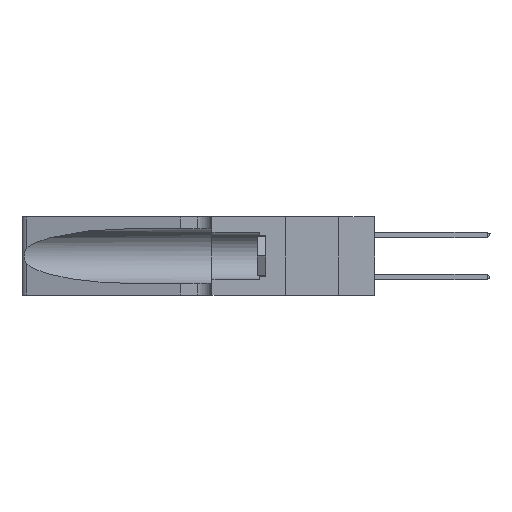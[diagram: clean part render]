
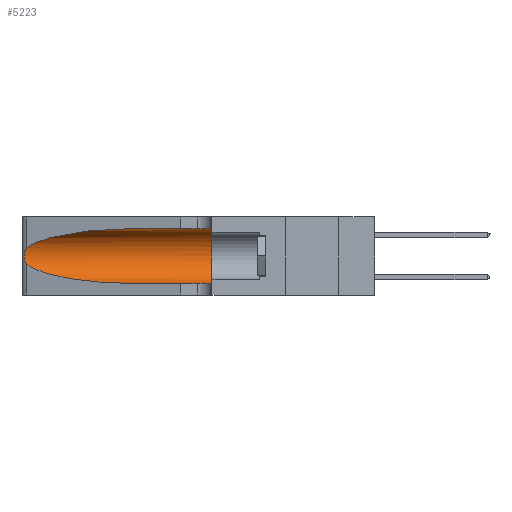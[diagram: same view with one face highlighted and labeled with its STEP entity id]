
A CAD part, left-side view. The second image highlights one B-rep face of the part: STEP entity #5223.
In plain terms, the highlighted cylindrical face has radius 3.308 mm (diameter 6.617 mm), a partial arc.
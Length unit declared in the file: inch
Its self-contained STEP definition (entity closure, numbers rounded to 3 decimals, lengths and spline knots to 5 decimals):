
#881 = CARTESIAN_POINT ( 'NONE',  ( 0.1305, 1.61858, 0.05475 ) ) ;
#1154 = EDGE_CURVE ( 'NONE', #2399, #32130, #8456, .T. ) ;
#1244 = ORIENTED_EDGE ( 'NONE', *, *, #23705, .T. ) ;
#1579 =( BOUNDED_CURVE ( )  B_SPLINE_CURVE ( 3, ( #5266, #29837, #29720, #38854 ),
 .UNSPECIFIED., .F., .F. ) 
 B_SPLINE_CURVE_WITH_KNOTS ( ( 4, 4 ),
 ( 1.5708, 2.84003 ),
 .UNSPECIFIED. ) 
 CURVE ( )  GEOMETRIC_REPRESENTATION_ITEM ( )  RATIONAL_B_SPLINE_CURVE ( ( 1., 0.87, 0.87, 1. ) ) 
 REPRESENTATION_ITEM ( '' )  );
#1945 = CARTESIAN_POINT ( 'NONE',  ( 0.26018, 1.23835, 0.19895 ) ) ;
#2399 = VERTEX_POINT ( 'NONE', #8929 ) ;
#2957 = ORIENTED_EDGE ( 'NONE', *, *, #26827, .T. ) ;
#3782 = EDGE_CURVE ( 'NONE', #24122, #13965, #1579, .T. ) ;
#3819 = VERTEX_POINT ( 'NONE', #29174 ) ;
#4473 = DIRECTION ( 'NONE',  ( 0., -1., 0. ) ) ;
#5223 = ADVANCED_FACE ( 'NONE', ( #20874 ), #28402, .F. ) ;
#5266 = CARTESIAN_POINT ( 'NONE',  ( 0.1305, 0.72297, 0.31525 ) ) ;
#5659 = CARTESIAN_POINT ( 'NONE',  ( 0.2373, 1.15595, 0.08982 ) ) ;
#6917 = DIRECTION ( 'NONE',  ( 0., 1., 0. ) ) ;
#7857 = VECTOR ( 'NONE', #20168, 39.37008 ) ;
#7904 = CARTESIAN_POINT ( 'NONE',  ( 0.26075, 1.23896, 0.178 ) ) ;
#8456 = CIRCLE ( 'NONE', #23205, 0.13025 ) ;
#8870 = CARTESIAN_POINT ( 'NONE',  ( 0.25487, 1.22718, 0.14631 ) ) ;
#8929 = CARTESIAN_POINT ( 'NONE',  ( 0.1305, 0.35, 0.31525 ) ) ;
#9087 = CARTESIAN_POINT ( 'NONE',  ( 0.1305, 0.72297, 0.05475 ) ) ;
#9824 = B_SPLINE_CURVE_WITH_KNOTS ( 'NONE', 3,
 ( #29441, #16912, #25865, #32092, #11217, #1945, #26258, #7904, #38062, #14008, #14292, #17045, #35158, #17284 ),
 .UNSPECIFIED., .F., .F.,
 ( 4, 2, 2, 2, 2, 2, 4 ),
 ( 0., 0.00027, 0.00053, 0.00107, 0.0016, 0.00187, 0.00214 ),
 .UNSPECIFIED. ) ;
#9852 = LINE ( 'NONE', #881, #33046 ) ;
#11217 = CARTESIAN_POINT ( 'NONE',  ( 0.25854, 1.2359, 0.20912 ) ) ;
#11310 = CARTESIAN_POINT ( 'NONE',  ( 0.1305, 1.61858, 0.31525 ) ) ;
#13034 = CARTESIAN_POINT ( 'NONE',  ( 0.1305, 0.72297, 0.31525 ) ) ;
#13965 = VERTEX_POINT ( 'NONE', #22958 ) ;
#14008 = CARTESIAN_POINT ( 'NONE',  ( 0.25856, 1.23593, 0.16098 ) ) ;
#14292 = CARTESIAN_POINT ( 'NONE',  ( 0.25789, 1.23486, 0.15765 ) ) ;
#14715 =( BOUNDED_CURVE ( )  B_SPLINE_CURVE ( 3, ( #29947, #5659, #16921, #9087 ),
 .UNSPECIFIED., .F., .T. ) 
 B_SPLINE_CURVE_WITH_KNOTS ( ( 4, 4 ),
 ( 3.44316, 4.71239 ),
 .UNSPECIFIED. ) 
 CURVE ( )  GEOMETRIC_REPRESENTATION_ITEM ( )  RATIONAL_B_SPLINE_CURVE ( ( 1., 0.87, 0.87, 1. ) ) 
 REPRESENTATION_ITEM ( '' )  );
#15980 = EDGE_CURVE ( 'NONE', #24122, #2399, #36723, .T. ) ;
#16296 = ORIENTED_EDGE ( 'NONE', *, *, #15980, .F. ) ;
#16912 = CARTESIAN_POINT ( 'NONE',  ( 0.25555, 1.22994, 0.2215 ) ) ;
#16921 = CARTESIAN_POINT ( 'NONE',  ( 0.18966, 0.96281, 0.05475 ) ) ;
#17045 = CARTESIAN_POINT ( 'NONE',  ( 0.25639, 1.23186, 0.15144 ) ) ;
#17284 = CARTESIAN_POINT ( 'NONE',  ( 0.25487, 1.22718, 0.14631 ) ) ;
#17561 = CARTESIAN_POINT ( 'NONE',  ( 0.1305, 0.35, 0.185 ) ) ;
#20168 = DIRECTION ( 'NONE',  ( 0., -1., 0. ) ) ;
#20874 = FACE_OUTER_BOUND ( 'NONE', #35509, .T. ) ;
#21376 = VERTEX_POINT ( 'NONE', #8870 ) ;
#22958 = CARTESIAN_POINT ( 'NONE',  ( 0.25487, 1.22718, 0.22369 ) ) ;
#23205 = AXIS2_PLACEMENT_3D ( 'NONE', #17561, #6917, #34150 ) ;
#23705 = EDGE_CURVE ( 'NONE', #13965, #21376, #9824, .T. ) ;
#24122 = VERTEX_POINT ( 'NONE', #13034 ) ;
#25865 = CARTESIAN_POINT ( 'NONE',  ( 0.25639, 1.23184, 0.21858 ) ) ;
#26258 = CARTESIAN_POINT ( 'NONE',  ( 0.26075, 1.23896, 0.19203 ) ) ;
#26827 = EDGE_CURVE ( 'NONE', #21376, #3819, #14715, .T. ) ;
#28037 = ORIENTED_EDGE ( 'NONE', *, *, #31503, .T. ) ;
#28402 = CYLINDRICAL_SURFACE ( 'NONE', #30828, 0.13025 ) ;
#29174 = CARTESIAN_POINT ( 'NONE',  ( 0.1305, 0.72297, 0.05475 ) ) ;
#29441 = CARTESIAN_POINT ( 'NONE',  ( 0.25487, 1.22718, 0.22369 ) ) ;
#29720 = CARTESIAN_POINT ( 'NONE',  ( 0.2373, 1.15595, 0.28018 ) ) ;
#29837 = CARTESIAN_POINT ( 'NONE',  ( 0.18966, 0.96281, 0.31525 ) ) ;
#29947 = CARTESIAN_POINT ( 'NONE',  ( 0.25487, 1.22718, 0.14631 ) ) ;
#30828 = AXIS2_PLACEMENT_3D ( 'NONE', #37696, #4473, #31719 ) ;
#31025 = DIRECTION ( 'NONE',  ( 0., -1., 0. ) ) ;
#31503 = EDGE_CURVE ( 'NONE', #3819, #32130, #9852, .T. ) ;
#31719 = DIRECTION ( 'NONE',  ( 0., 0., -1. ) ) ;
#32092 = CARTESIAN_POINT ( 'NONE',  ( 0.25787, 1.23484, 0.2124 ) ) ;
#32130 = VERTEX_POINT ( 'NONE', #36842 ) ;
#33046 = VECTOR ( 'NONE', #31025, 39.37008 ) ;
#34150 = DIRECTION ( 'NONE',  ( 0., 0., 1. ) ) ;
#34380 = ORIENTED_EDGE ( 'NONE', *, *, #1154, .F. ) ;
#35158 = CARTESIAN_POINT ( 'NONE',  ( 0.25555, 1.22993, 0.14849 ) ) ;
#35509 = EDGE_LOOP ( 'NONE', ( #38660, #1244, #2957, #28037, #34380, #16296 ) ) ;
#36723 = LINE ( 'NONE', #11310, #7857 ) ;
#36842 = CARTESIAN_POINT ( 'NONE',  ( 0.1305, 0.35, 0.05475 ) ) ;
#37696 = CARTESIAN_POINT ( 'NONE',  ( 0.1305, 1.61858, 0.185 ) ) ;
#38062 = CARTESIAN_POINT ( 'NONE',  ( 0.26017, 1.23833, 0.17102 ) ) ;
#38660 = ORIENTED_EDGE ( 'NONE', *, *, #3782, .T. ) ;
#38854 = CARTESIAN_POINT ( 'NONE',  ( 0.25487, 1.22718, 0.22369 ) ) ;
